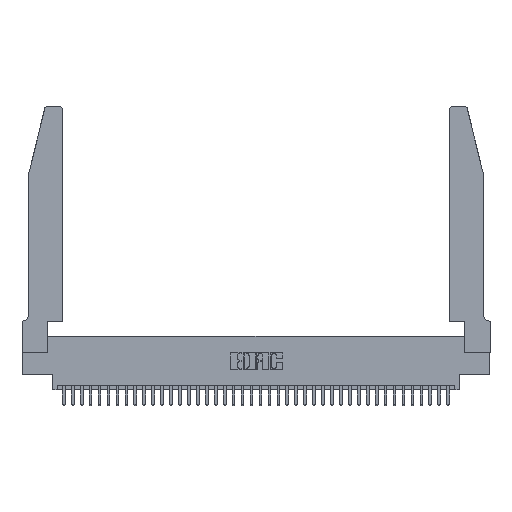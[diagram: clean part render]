
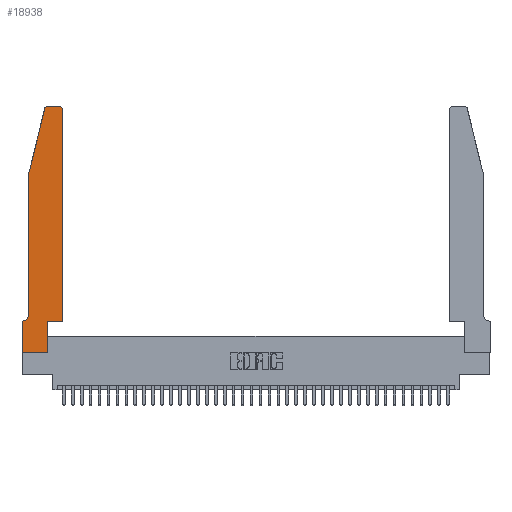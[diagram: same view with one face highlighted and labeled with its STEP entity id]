
A CAD part, top view. The second image highlights one B-rep face of the part: STEP entity #18938.
In plain terms, the highlighted planar face has unit normal (0, 0, 1).
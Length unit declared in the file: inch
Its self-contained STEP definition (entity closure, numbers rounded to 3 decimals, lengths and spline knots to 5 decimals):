
#97 = CARTESIAN_POINT ( 'NONE',  ( 0.2605, 2.75, 0.37 ) ) ;
#322 = VECTOR ( 'NONE', #5212, 39.37008 ) ;
#1175 = AXIS2_PLACEMENT_3D ( 'NONE', #30726, #30212, #18417 ) ;
#1371 = DIRECTION ( 'NONE',  ( -1., 0., 0. ) ) ;
#1576 = VERTEX_POINT ( 'NONE', #28712 ) ;
#1869 = CARTESIAN_POINT ( 'NONE',  ( 0., 0., 0.37 ) ) ;
#2890 = VERTEX_POINT ( 'NONE', #31980 ) ;
#3763 = VERTEX_POINT ( 'NONE', #6676 ) ;
#4709 = CIRCLE ( 'NONE', #25066, 0.07 ) ;
#4800 = VECTOR ( 'NONE', #11782, 39.37008 ) ;
#5017 = CARTESIAN_POINT ( 'NONE',  ( 0.284, 2.72, 0.37 ) ) ;
#5212 = DIRECTION ( 'NONE',  ( 1., 0., 0. ) ) ;
#5228 = EDGE_CURVE ( 'NONE', #39041, #31382, #37017, .T. ) ;
#5407 = VERTEX_POINT ( 'NONE', #37139 ) ;
#6105 = ORIENTED_EDGE ( 'NONE', *, *, #23573, .T. ) ;
#6676 = CARTESIAN_POINT ( 'NONE',  ( 0., 0., 0.37 ) ) ;
#7244 = LINE ( 'NONE', #31538, #17716 ) ;
#7581 = LINE ( 'NONE', #23743, #27076 ) ;
#7774 = EDGE_CURVE ( 'NONE', #1576, #8940, #24907, .T. ) ;
#8376 = AXIS2_PLACEMENT_3D ( 'NONE', #5017, #11207, #17485 ) ;
#8940 = VERTEX_POINT ( 'NONE', #35262 ) ;
#9023 = CARTESIAN_POINT ( 'NONE',  ( 0.0755, 2., 0.37 ) ) ;
#9360 = CARTESIAN_POINT ( 'NONE',  ( 0.25487, 2.72718, 0.37 ) ) ;
#9669 = EDGE_CURVE ( 'NONE', #18424, #1576, #11402, .T. ) ;
#9734 = CARTESIAN_POINT ( 'NONE',  ( 0.4505, 0.35, 0.37 ) ) ;
#10603 = EDGE_CURVE ( 'NONE', #15621, #39041, #4709, .T. ) ;
#10946 = VECTOR ( 'NONE', #21319, 39.37008 ) ;
#11207 = DIRECTION ( 'NONE',  ( 0., 0., 1. ) ) ;
#11402 = LINE ( 'NONE', #14844, #4800 ) ;
#11691 = DIRECTION ( 'NONE',  ( -0.239, -0.971, 0. ) ) ;
#11782 = DIRECTION ( 'NONE',  ( 0., 1., 0. ) ) ;
#12926 = EDGE_CURVE ( 'NONE', #5407, #34559, #18729, .T. ) ;
#13482 = CARTESIAN_POINT ( 'NONE',  ( 0.0755, 0.42, 0.37 ) ) ;
#13793 = CARTESIAN_POINT ( 'NONE',  ( 0.0055, 0.42, 0.37 ) ) ;
#14844 = CARTESIAN_POINT ( 'NONE',  ( 0.4505, 0.35, 0.37 ) ) ;
#15211 = ORIENTED_EDGE ( 'NONE', *, *, #34726, .T. ) ;
#15419 = LINE ( 'NONE', #38648, #32493 ) ;
#15621 = VERTEX_POINT ( 'NONE', #13482 ) ;
#15888 = DIRECTION ( 'NONE',  ( 0., 0., 1. ) ) ;
#15968 = ORIENTED_EDGE ( 'NONE', *, *, #5228, .T. ) ;
#16349 = VERTEX_POINT ( 'NONE', #29716 ) ;
#16851 = ORIENTED_EDGE ( 'NONE', *, *, #21914, .T. ) ;
#17022 = CARTESIAN_POINT ( 'NONE',  ( 0.0055, 0.35, 0.37 ) ) ;
#17129 = EDGE_LOOP ( 'NONE', ( #15211, #25819, #16851, #31566, #23023, #15968, #22556, #6105, #23451, #25795, #33422, #22641 ) ) ;
#17304 = CARTESIAN_POINT ( 'NONE',  ( 0.0755, 2., 0.37 ) ) ;
#17485 = DIRECTION ( 'NONE',  ( 1., 0., 0. ) ) ;
#17716 = VECTOR ( 'NONE', #34988, 39.37008 ) ;
#18417 = DIRECTION ( 'NONE',  ( 1., 0., 0. ) ) ;
#18424 = VERTEX_POINT ( 'NONE', #34390 ) ;
#18665 = DIRECTION ( 'NONE',  ( 1., 0., 0. ) ) ;
#18729 = CIRCLE ( 'NONE', #8376, 0.03 ) ;
#18905 = DIRECTION ( 'NONE',  ( 1., 0., 0. ) ) ;
#18938 = ADVANCED_FACE ( 'NONE', ( #35407 ), #24364, .T. ) ;
#20901 = VECTOR ( 'NONE', #18905, 39.37008 ) ;
#21319 = DIRECTION ( 'NONE',  ( -1., 0., 0. ) ) ;
#21914 = EDGE_CURVE ( 'NONE', #34559, #27970, #7581, .T. ) ;
#22556 = ORIENTED_EDGE ( 'NONE', *, *, #35072, .T. ) ;
#22641 = ORIENTED_EDGE ( 'NONE', *, *, #7774, .T. ) ;
#23023 = ORIENTED_EDGE ( 'NONE', *, *, #10603, .T. ) ;
#23202 = DIRECTION ( 'NONE',  ( -1., 0., 0. ) ) ;
#23451 = ORIENTED_EDGE ( 'NONE', *, *, #26347, .T. ) ;
#23573 = EDGE_CURVE ( 'NONE', #3763, #16349, #23605, .T. ) ;
#23605 = LINE ( 'NONE', #1869, #322 ) ;
#23722 = CARTESIAN_POINT ( 'NONE',  ( 0.0755, 0.35, 0.37 ) ) ;
#23743 = CARTESIAN_POINT ( 'NONE',  ( 0.0755, 2., 0.37 ) ) ;
#23942 = DIRECTION ( 'NONE',  ( 0., -1., 0. ) ) ;
#23972 = VECTOR ( 'NONE', #1371, 39.37008 ) ;
#24364 = PLANE ( 'NONE',  #1175 ) ;
#24671 = EDGE_CURVE ( 'NONE', #27970, #15621, #28760, .T. ) ;
#24686 = LINE ( 'NONE', #9734, #20901 ) ;
#24907 = CIRCLE ( 'NONE', #38494, 0.03 ) ;
#25007 = CARTESIAN_POINT ( 'NONE',  ( 0.4205, 2.72, 0.37 ) ) ;
#25066 = AXIS2_PLACEMENT_3D ( 'NONE', #13793, #25611, #23202 ) ;
#25611 = DIRECTION ( 'NONE',  ( 0., 0., -1. ) ) ;
#25795 = ORIENTED_EDGE ( 'NONE', *, *, #38260, .T. ) ;
#25819 = ORIENTED_EDGE ( 'NONE', *, *, #12926, .T. ) ;
#26347 = EDGE_CURVE ( 'NONE', #16349, #2890, #7244, .T. ) ;
#27076 = VECTOR ( 'NONE', #11691, 39.37008 ) ;
#27970 = VERTEX_POINT ( 'NONE', #17304 ) ;
#28231 = LINE ( 'NONE', #97, #23972 ) ;
#28712 = CARTESIAN_POINT ( 'NONE',  ( 0.4505, 2.72, 0.37 ) ) ;
#28760 = LINE ( 'NONE', #9023, #29229 ) ;
#29229 = VECTOR ( 'NONE', #36447, 39.37008 ) ;
#29716 = CARTESIAN_POINT ( 'NONE',  ( 0.2865, 0., 0.37 ) ) ;
#30155 = CARTESIAN_POINT ( 'NONE',  ( 0., 0.35, 0.37 ) ) ;
#30212 = DIRECTION ( 'NONE',  ( 0., 0., 1. ) ) ;
#30726 = CARTESIAN_POINT ( 'NONE',  ( 0., 0.35, 0.37 ) ) ;
#31382 = VERTEX_POINT ( 'NONE', #30155 ) ;
#31538 = CARTESIAN_POINT ( 'NONE',  ( 0.2865, 0.35, 0.37 ) ) ;
#31566 = ORIENTED_EDGE ( 'NONE', *, *, #24671, .T. ) ;
#31980 = CARTESIAN_POINT ( 'NONE',  ( 0.2865, 0.35, 0.37 ) ) ;
#32493 = VECTOR ( 'NONE', #23942, 39.37008 ) ;
#33422 = ORIENTED_EDGE ( 'NONE', *, *, #9669, .T. ) ;
#34390 = CARTESIAN_POINT ( 'NONE',  ( 0.4505, 0.35, 0.37 ) ) ;
#34559 = VERTEX_POINT ( 'NONE', #9360 ) ;
#34726 = EDGE_CURVE ( 'NONE', #8940, #5407, #28231, .T. ) ;
#34988 = DIRECTION ( 'NONE',  ( 0., 1., 0. ) ) ;
#35072 = EDGE_CURVE ( 'NONE', #31382, #3763, #15419, .T. ) ;
#35262 = CARTESIAN_POINT ( 'NONE',  ( 0.4205, 2.75, 0.37 ) ) ;
#35407 = FACE_OUTER_BOUND ( 'NONE', #17129, .T. ) ;
#36447 = DIRECTION ( 'NONE',  ( 0., -1., 0. ) ) ;
#37017 = LINE ( 'NONE', #23722, #10946 ) ;
#37139 = CARTESIAN_POINT ( 'NONE',  ( 0.284, 2.75, 0.37 ) ) ;
#38260 = EDGE_CURVE ( 'NONE', #2890, #18424, #24686, .T. ) ;
#38494 = AXIS2_PLACEMENT_3D ( 'NONE', #25007, #15888, #18665 ) ;
#38648 = CARTESIAN_POINT ( 'NONE',  ( 0., 0., 0.37 ) ) ;
#39041 = VERTEX_POINT ( 'NONE', #17022 ) ;
